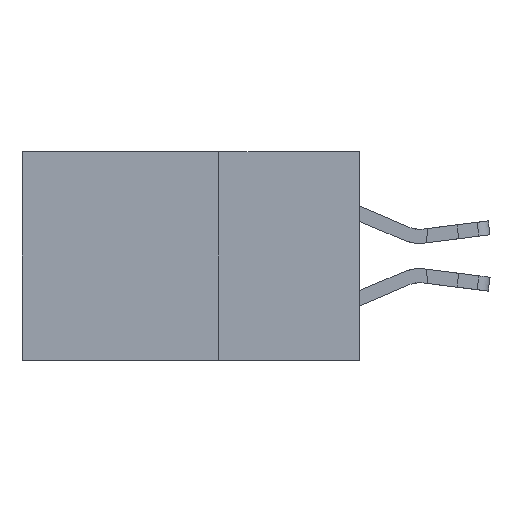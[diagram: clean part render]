
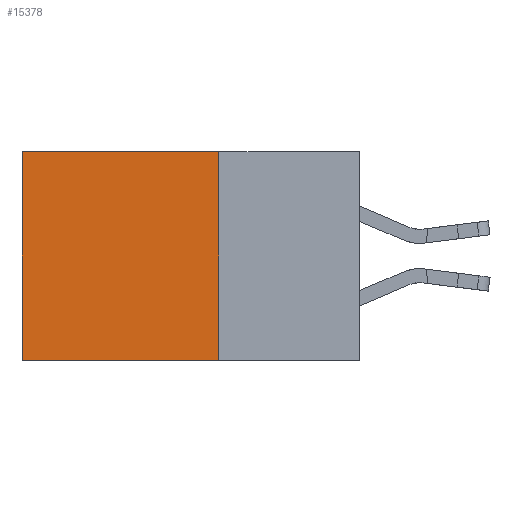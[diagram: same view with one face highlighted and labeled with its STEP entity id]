
A CAD part, left-side view. The second image highlights one B-rep face of the part: STEP entity #15378.
In plain terms, the highlighted planar face has unit normal (-1, 0, 0).
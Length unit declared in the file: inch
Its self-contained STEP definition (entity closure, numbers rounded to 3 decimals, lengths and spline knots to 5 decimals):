
#726 = DIRECTION ( 'NONE',  ( 0., 0., -1. ) ) ;
#1491 = LINE ( 'NONE', #2028, #16601 ) ;
#2028 = CARTESIAN_POINT ( 'NONE',  ( 0.2875, 0.25, 0. ) ) ;
#2430 = ORIENTED_EDGE ( 'NONE', *, *, #18854, .T. ) ;
#2491 = DIRECTION ( 'NONE',  ( 1., 0., 0. ) ) ;
#2754 = LINE ( 'NONE', #17149, #10272 ) ;
#3438 = AXIS2_PLACEMENT_3D ( 'NONE', #12765, #2491, #12828 ) ;
#3716 = FACE_OUTER_BOUND ( 'NONE', #12178, .T. ) ;
#3792 = VECTOR ( 'NONE', #4357, 39.37008 ) ;
#4170 = CARTESIAN_POINT ( 'NONE',  ( 0.2875, 0.6, 0. ) ) ;
#4357 = DIRECTION ( 'NONE',  ( 0., 1., 0. ) ) ;
#4585 = CARTESIAN_POINT ( 'NONE',  ( 0.2875, 0.25, -0.37 ) ) ;
#4782 = EDGE_CURVE ( 'NONE', #7549, #13208, #7794, .T. ) ;
#5366 = CARTESIAN_POINT ( 'NONE',  ( 0.2875, 0.6, 0. ) ) ;
#5774 = EDGE_CURVE ( 'NONE', #15268, #7549, #2754, .T. ) ;
#7163 = ORIENTED_EDGE ( 'NONE', *, *, #4782, .F. ) ;
#7549 = VERTEX_POINT ( 'NONE', #8462 ) ;
#7794 = LINE ( 'NONE', #4585, #3792 ) ;
#8462 = CARTESIAN_POINT ( 'NONE',  ( 0.2875, 0.25, -0.37 ) ) ;
#8472 = EDGE_CURVE ( 'NONE', #10357, #13208, #17116, .T. ) ;
#9995 = PLANE ( 'NONE',  #3438 ) ;
#10272 = VECTOR ( 'NONE', #15743, 39.37008 ) ;
#10357 = VERTEX_POINT ( 'NONE', #4170 ) ;
#11163 = CARTESIAN_POINT ( 'NONE',  ( 0.2875, 0.25, 0. ) ) ;
#12178 = EDGE_LOOP ( 'NONE', ( #17797, #7163, #13437, #2430 ) ) ;
#12498 = DIRECTION ( 'NONE',  ( 0., 1., 0. ) ) ;
#12765 = CARTESIAN_POINT ( 'NONE',  ( 0.2875, 0.25, 0. ) ) ;
#12828 = DIRECTION ( 'NONE',  ( 0., 0., -1. ) ) ;
#13208 = VERTEX_POINT ( 'NONE', #18996 ) ;
#13437 = ORIENTED_EDGE ( 'NONE', *, *, #5774, .F. ) ;
#15268 = VERTEX_POINT ( 'NONE', #11163 ) ;
#15378 = ADVANCED_FACE ( 'NONE', ( #3716 ), #9995, .F. ) ;
#15743 = DIRECTION ( 'NONE',  ( 0., 0., -1. ) ) ;
#16252 = VECTOR ( 'NONE', #726, 39.37008 ) ;
#16601 = VECTOR ( 'NONE', #12498, 39.37008 ) ;
#17116 = LINE ( 'NONE', #5366, #16252 ) ;
#17149 = CARTESIAN_POINT ( 'NONE',  ( 0.2875, 0.25, 0. ) ) ;
#17797 = ORIENTED_EDGE ( 'NONE', *, *, #8472, .T. ) ;
#18854 = EDGE_CURVE ( 'NONE', #15268, #10357, #1491, .T. ) ;
#18996 = CARTESIAN_POINT ( 'NONE',  ( 0.2875, 0.6, -0.37 ) ) ;
